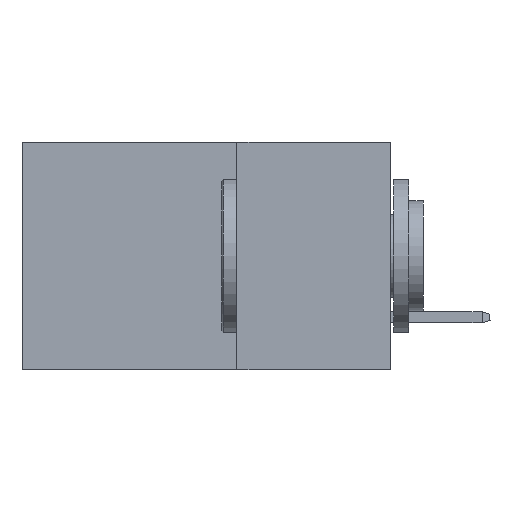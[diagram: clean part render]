
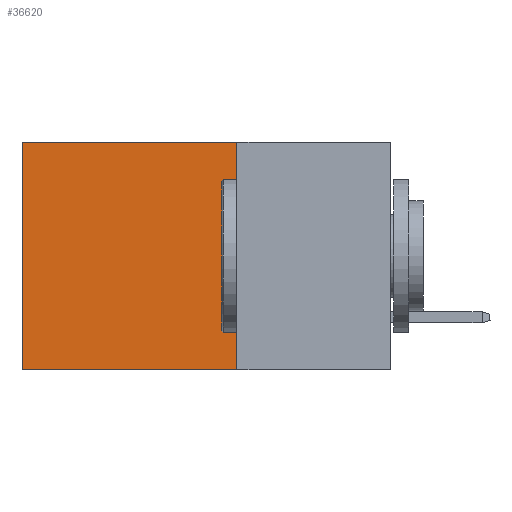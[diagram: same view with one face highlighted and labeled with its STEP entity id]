
A CAD part, left-side view. The second image highlights one B-rep face of the part: STEP entity #36620.
In plain terms, the highlighted planar face has unit normal (-1, 0, 0).
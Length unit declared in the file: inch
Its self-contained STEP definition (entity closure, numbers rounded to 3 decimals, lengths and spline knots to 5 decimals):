
#637 = PLANE ( 'NONE',  #25523 ) ;
#2425 = CARTESIAN_POINT ( 'NONE',  ( 0.2875, 0.25, 0. ) ) ;
#4513 = LINE ( 'NONE', #43709, #31302 ) ;
#4666 = DIRECTION ( 'NONE',  ( 0., 1., 0. ) ) ;
#7139 = VERTEX_POINT ( 'NONE', #13628 ) ;
#9921 = CARTESIAN_POINT ( 'NONE',  ( 0.2875, 0.25, 0. ) ) ;
#11977 = CARTESIAN_POINT ( 'NONE',  ( 0.2875, 0.25, -0.37 ) ) ;
#13628 = CARTESIAN_POINT ( 'NONE',  ( 0.2875, 0.6, -0.37 ) ) ;
#14533 = ORIENTED_EDGE ( 'NONE', *, *, #43653, .F. ) ;
#16217 = ORIENTED_EDGE ( 'NONE', *, *, #35891, .F. ) ;
#16795 = VECTOR ( 'NONE', #44642, 39.37008 ) ;
#17989 = LINE ( 'NONE', #44372, #36584 ) ;
#18117 = CARTESIAN_POINT ( 'NONE',  ( 0.2875, 0.25, 0. ) ) ;
#20335 = DIRECTION ( 'NONE',  ( 0., 0., -1. ) ) ;
#21897 = DIRECTION ( 'NONE',  ( 0., 0., -1. ) ) ;
#22802 = EDGE_CURVE ( 'NONE', #29729, #7139, #4513, .T. ) ;
#24925 = LINE ( 'NONE', #9921, #16795 ) ;
#25523 = AXIS2_PLACEMENT_3D ( 'NONE', #18117, #31804, #21897 ) ;
#26135 = ORIENTED_EDGE ( 'NONE', *, *, #22802, .T. ) ;
#29729 = VERTEX_POINT ( 'NONE', #44010 ) ;
#29850 = CARTESIAN_POINT ( 'NONE',  ( 0.2875, 0.25, -0.37 ) ) ;
#31248 = VERTEX_POINT ( 'NONE', #29850 ) ;
#31302 = VECTOR ( 'NONE', #39596, 39.37008 ) ;
#31804 = DIRECTION ( 'NONE',  ( 1., 0., 0. ) ) ;
#32588 = VECTOR ( 'NONE', #4666, 39.37008 ) ;
#35443 = LINE ( 'NONE', #11977, #32588 ) ;
#35891 = EDGE_CURVE ( 'NONE', #31248, #7139, #35443, .T. ) ;
#36031 = EDGE_LOOP ( 'NONE', ( #26135, #16217, #14533, #40439 ) ) ;
#36584 = VECTOR ( 'NONE', #20335, 39.37008 ) ;
#36620 = ADVANCED_FACE ( 'NONE', ( #40931 ), #637, .F. ) ;
#39596 = DIRECTION ( 'NONE',  ( 0., 0., -1. ) ) ;
#40439 = ORIENTED_EDGE ( 'NONE', *, *, #45046, .T. ) ;
#40931 = FACE_OUTER_BOUND ( 'NONE', #36031, .T. ) ;
#42003 = VERTEX_POINT ( 'NONE', #2425 ) ;
#43653 = EDGE_CURVE ( 'NONE', #42003, #31248, #17989, .T. ) ;
#43709 = CARTESIAN_POINT ( 'NONE',  ( 0.2875, 0.6, 0. ) ) ;
#44010 = CARTESIAN_POINT ( 'NONE',  ( 0.2875, 0.6, 0. ) ) ;
#44372 = CARTESIAN_POINT ( 'NONE',  ( 0.2875, 0.25, 0. ) ) ;
#44642 = DIRECTION ( 'NONE',  ( 0., 1., 0. ) ) ;
#45046 = EDGE_CURVE ( 'NONE', #42003, #29729, #24925, .T. ) ;
